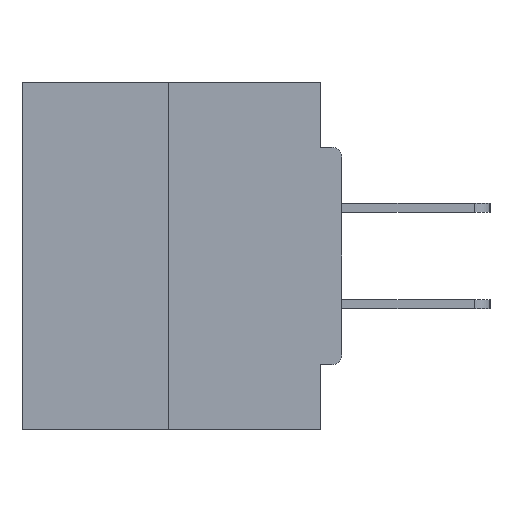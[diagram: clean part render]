
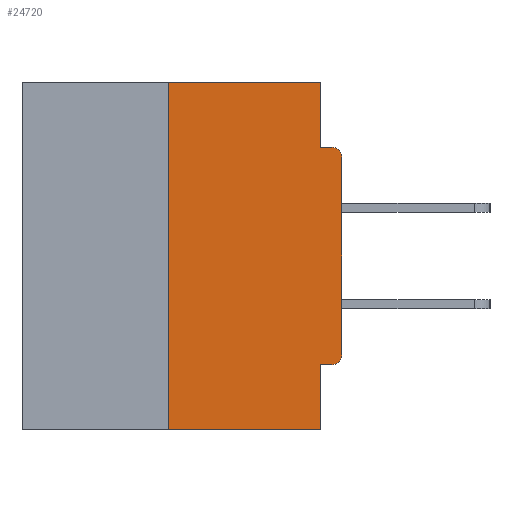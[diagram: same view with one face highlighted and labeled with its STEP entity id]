
A CAD part, left-side view. The second image highlights one B-rep face of the part: STEP entity #24720.
In plain terms, the highlighted planar face has unit normal (-1, 0, 0).
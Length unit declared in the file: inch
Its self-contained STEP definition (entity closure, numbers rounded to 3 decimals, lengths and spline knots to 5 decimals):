
#565 = EDGE_CURVE ( 'NONE', #26823, #14042, #13986, .T. ) ;
#880 = LINE ( 'NONE', #23823, #24494 ) ;
#1028 = VERTEX_POINT ( 'NONE', #11554 ) ;
#1584 = LINE ( 'NONE', #5061, #2422 ) ;
#2035 = VERTEX_POINT ( 'NONE', #26996 ) ;
#2422 = VECTOR ( 'NONE', #13307, 39.37008 ) ;
#3364 = DIRECTION ( 'NONE',  ( 0., 0., 1. ) ) ;
#3924 = DIRECTION ( 'NONE',  ( 0., 0., -1. ) ) ;
#4025 = ORIENTED_EDGE ( 'NONE', *, *, #26505, .F. ) ;
#4175 = VERTEX_POINT ( 'NONE', #29911 ) ;
#4294 = PLANE ( 'NONE',  #14153 ) ;
#4969 = LINE ( 'NONE', #11924, #23979 ) ;
#5061 = CARTESIAN_POINT ( 'NONE',  ( 0., 0.46, 0. ) ) ;
#5546 = LINE ( 'NONE', #24952, #7247 ) ;
#5763 = CARTESIAN_POINT ( 'NONE',  ( 0., 0.031, -0.5 ) ) ;
#6581 = CARTESIAN_POINT ( 'NONE',  ( 0., 0.031, 0. ) ) ;
#6769 = CARTESIAN_POINT ( 'NONE',  ( 0., 0.031, 0. ) ) ;
#6819 = VECTOR ( 'NONE', #25724, 39.37008 ) ;
#7098 = ORIENTED_EDGE ( 'NONE', *, *, #34974, .F. ) ;
#7116 = DIRECTION ( 'NONE',  ( 1., 0., 0. ) ) ;
#7247 = VECTOR ( 'NONE', #33135, 39.37008 ) ;
#7359 = ORIENTED_EDGE ( 'NONE', *, *, #565, .F. ) ;
#8090 = LINE ( 'NONE', #12645, #22040 ) ;
#8373 = EDGE_CURVE ( 'NONE', #13555, #10150, #8090, .T. ) ;
#10150 = VERTEX_POINT ( 'NONE', #18331 ) ;
#10448 = VECTOR ( 'NONE', #20856, 39.37008 ) ;
#10554 = CARTESIAN_POINT ( 'NONE',  ( 0., 0.25, -0.5 ) ) ;
#10579 = ORIENTED_EDGE ( 'NONE', *, *, #17669, .T. ) ;
#10607 = DIRECTION ( 'NONE',  ( 0., 0., -1. ) ) ;
#11554 = CARTESIAN_POINT ( 'NONE',  ( 0., 0.015, -0.0935 ) ) ;
#11924 = CARTESIAN_POINT ( 'NONE',  ( 0., 0.031, -0.5 ) ) ;
#11952 = DIRECTION ( 'NONE',  ( 0., 0., -1. ) ) ;
#12645 = CARTESIAN_POINT ( 'NONE',  ( 0., 0., -0.4065 ) ) ;
#13307 = DIRECTION ( 'NONE',  ( 0., -1., 0. ) ) ;
#13555 = VERTEX_POINT ( 'NONE', #33852 ) ;
#13583 = VERTEX_POINT ( 'NONE', #26497 ) ;
#13986 = LINE ( 'NONE', #6581, #6819 ) ;
#14042 = VERTEX_POINT ( 'NONE', #28072 ) ;
#14153 = AXIS2_PLACEMENT_3D ( 'NONE', #28771, #7116, #25927 ) ;
#14531 = ORIENTED_EDGE ( 'NONE', *, *, #8373, .F. ) ;
#14583 = CARTESIAN_POINT ( 'NONE',  ( 0., 0., -0.0935 ) ) ;
#14912 = CARTESIAN_POINT ( 'NONE',  ( 0., 0.015, -0.1085 ) ) ;
#15846 = ORIENTED_EDGE ( 'NONE', *, *, #19980, .T. ) ;
#15865 = AXIS2_PLACEMENT_3D ( 'NONE', #14912, #22946, #11952 ) ;
#16014 = ORIENTED_EDGE ( 'NONE', *, *, #19065, .T. ) ;
#17669 = EDGE_CURVE ( 'NONE', #13555, #13583, #19659, .T. ) ;
#18127 = DIRECTION ( 'NONE',  ( 0., 1., 0. ) ) ;
#18160 = CARTESIAN_POINT ( 'NONE',  ( 0., 0.25, 0. ) ) ;
#18331 = CARTESIAN_POINT ( 'NONE',  ( 0., 0.031, -0.4065 ) ) ;
#18800 = VERTEX_POINT ( 'NONE', #5763 ) ;
#19065 = EDGE_CURVE ( 'NONE', #2035, #1028, #28443, .T. ) ;
#19165 = EDGE_CURVE ( 'NONE', #23212, #18800, #5546, .T. ) ;
#19659 = CIRCLE ( 'NONE', #32411, 0.015 ) ;
#19980 = EDGE_CURVE ( 'NONE', #13583, #2035, #880, .T. ) ;
#20856 = DIRECTION ( 'NONE',  ( 0., 0., 1. ) ) ;
#21497 = DIRECTION ( 'NONE',  ( -1., 0., 0. ) ) ;
#21879 = ORIENTED_EDGE ( 'NONE', *, *, #19165, .T. ) ;
#21919 = ORIENTED_EDGE ( 'NONE', *, *, #34727, .F. ) ;
#22001 = EDGE_CURVE ( 'NONE', #14042, #1028, #25646, .T. ) ;
#22040 = VECTOR ( 'NONE', #18127, 39.37008 ) ;
#22437 = FACE_OUTER_BOUND ( 'NONE', #33845, .T. ) ;
#22946 = DIRECTION ( 'NONE',  ( -1., 0., 0. ) ) ;
#23212 = VERTEX_POINT ( 'NONE', #10554 ) ;
#23823 = CARTESIAN_POINT ( 'NONE',  ( 0., 0., 0. ) ) ;
#23979 = VECTOR ( 'NONE', #3924, 39.37008 ) ;
#24494 = VECTOR ( 'NONE', #3364, 39.37008 ) ;
#24720 = ADVANCED_FACE ( 'NONE', ( #22437 ), #4294, .F. ) ;
#24952 = CARTESIAN_POINT ( 'NONE',  ( 0., 0.46, -0.5 ) ) ;
#25000 = DIRECTION ( 'NONE',  ( 0., -1., 0. ) ) ;
#25646 = LINE ( 'NONE', #14583, #26491 ) ;
#25724 = DIRECTION ( 'NONE',  ( 0., 0., -1. ) ) ;
#25927 = DIRECTION ( 'NONE',  ( 0., 0., -1. ) ) ;
#26491 = VECTOR ( 'NONE', #25000, 39.37008 ) ;
#26497 = CARTESIAN_POINT ( 'NONE',  ( 0., 0., -0.3915 ) ) ;
#26505 = EDGE_CURVE ( 'NONE', #23212, #4175, #26969, .T. ) ;
#26572 = ORIENTED_EDGE ( 'NONE', *, *, #22001, .F. ) ;
#26823 = VERTEX_POINT ( 'NONE', #6769 ) ;
#26838 = CARTESIAN_POINT ( 'NONE',  ( 0., 0.015, -0.3915 ) ) ;
#26969 = LINE ( 'NONE', #18160, #10448 ) ;
#26996 = CARTESIAN_POINT ( 'NONE',  ( 0., 0., -0.1085 ) ) ;
#28072 = CARTESIAN_POINT ( 'NONE',  ( 0., 0.031, -0.0935 ) ) ;
#28443 = CIRCLE ( 'NONE', #15865, 0.015 ) ;
#28771 = CARTESIAN_POINT ( 'NONE',  ( 0., 0.46, 0. ) ) ;
#29911 = CARTESIAN_POINT ( 'NONE',  ( 0., 0.25, 0. ) ) ;
#32411 = AXIS2_PLACEMENT_3D ( 'NONE', #26838, #21497, #10607 ) ;
#33135 = DIRECTION ( 'NONE',  ( 0., -1., 0. ) ) ;
#33845 = EDGE_LOOP ( 'NONE', ( #7098, #4025, #21879, #21919, #14531, #10579, #15846, #16014, #26572, #7359 ) ) ;
#33852 = CARTESIAN_POINT ( 'NONE',  ( 0., 0.015, -0.4065 ) ) ;
#34727 = EDGE_CURVE ( 'NONE', #10150, #18800, #4969, .T. ) ;
#34974 = EDGE_CURVE ( 'NONE', #4175, #26823, #1584, .T. ) ;
